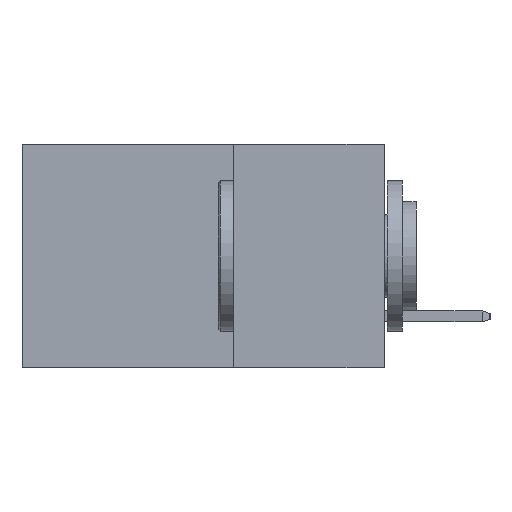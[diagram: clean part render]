
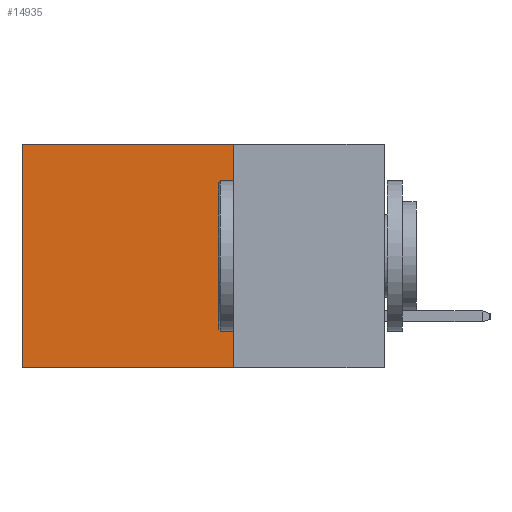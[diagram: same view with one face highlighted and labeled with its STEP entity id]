
A CAD part, left-side view. The second image highlights one B-rep face of the part: STEP entity #14935.
In plain terms, the highlighted planar face has unit normal (-1, 0, 0).
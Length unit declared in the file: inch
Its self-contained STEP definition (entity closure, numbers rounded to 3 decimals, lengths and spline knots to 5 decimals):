
#151 = LINE ( 'NONE', #11395, #6704 ) ;
#161 = CARTESIAN_POINT ( 'NONE',  ( 0.2615, 0.25, -0.37 ) ) ;
#330 = AXIS2_PLACEMENT_3D ( 'NONE', #2833, #9606, #14769 ) ;
#523 = FACE_OUTER_BOUND ( 'NONE', #8301, .T. ) ;
#1107 = VERTEX_POINT ( 'NONE', #6601 ) ;
#1608 = LINE ( 'NONE', #14158, #8453 ) ;
#1617 = EDGE_CURVE ( 'NONE', #1107, #13607, #12924, .T. ) ;
#2033 = DIRECTION ( 'NONE',  ( 0., 1., 0. ) ) ;
#2252 = DIRECTION ( 'NONE',  ( 0., 1., 0. ) ) ;
#2817 = CARTESIAN_POINT ( 'NONE',  ( 0.2615, 0.6, -0.37 ) ) ;
#2833 = CARTESIAN_POINT ( 'NONE',  ( 0.2615, 0.25, -0.37 ) ) ;
#2901 = LINE ( 'NONE', #161, #9686 ) ;
#3646 = CARTESIAN_POINT ( 'NONE',  ( 0.2615, 0.6, -0.37 ) ) ;
#3693 = ORIENTED_EDGE ( 'NONE', *, *, #1617, .T. ) ;
#3905 = EDGE_CURVE ( 'NONE', #14700, #13607, #1608, .T. ) ;
#5814 = EDGE_CURVE ( 'NONE', #13347, #1107, #151, .T. ) ;
#5972 = VECTOR ( 'NONE', #17135, 39.37008 ) ;
#6402 = CARTESIAN_POINT ( 'NONE',  ( 0.2615, 0.25, 0. ) ) ;
#6537 = ORIENTED_EDGE ( 'NONE', *, *, #3905, .F. ) ;
#6601 = CARTESIAN_POINT ( 'NONE',  ( 0.2615, 0.6, 0. ) ) ;
#6704 = VECTOR ( 'NONE', #2033, 39.37008 ) ;
#7346 = ORIENTED_EDGE ( 'NONE', *, *, #16473, .F. ) ;
#8301 = EDGE_LOOP ( 'NONE', ( #3693, #6537, #7346, #10849 ) ) ;
#8453 = VECTOR ( 'NONE', #2252, 39.37008 ) ;
#9606 = DIRECTION ( 'NONE',  ( 1., 0., 0. ) ) ;
#9686 = VECTOR ( 'NONE', #11038, 39.37008 ) ;
#10849 = ORIENTED_EDGE ( 'NONE', *, *, #5814, .T. ) ;
#11038 = DIRECTION ( 'NONE',  ( 0., 0., -1. ) ) ;
#11395 = CARTESIAN_POINT ( 'NONE',  ( 0.2615, 0.25, 0. ) ) ;
#12924 = LINE ( 'NONE', #3646, #5972 ) ;
#13347 = VERTEX_POINT ( 'NONE', #6402 ) ;
#13472 = PLANE ( 'NONE',  #330 ) ;
#13607 = VERTEX_POINT ( 'NONE', #2817 ) ;
#14158 = CARTESIAN_POINT ( 'NONE',  ( 0.2615, 0.25, -0.37 ) ) ;
#14270 = CARTESIAN_POINT ( 'NONE',  ( 0.2615, 0.25, -0.37 ) ) ;
#14700 = VERTEX_POINT ( 'NONE', #14270 ) ;
#14769 = DIRECTION ( 'NONE',  ( 0., 0., -1. ) ) ;
#14935 = ADVANCED_FACE ( 'NONE', ( #523 ), #13472, .F. ) ;
#16473 = EDGE_CURVE ( 'NONE', #13347, #14700, #2901, .T. ) ;
#17135 = DIRECTION ( 'NONE',  ( 0., 0., -1. ) ) ;
